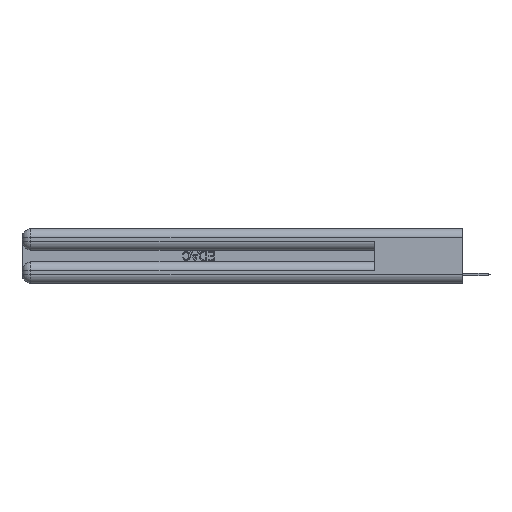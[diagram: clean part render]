
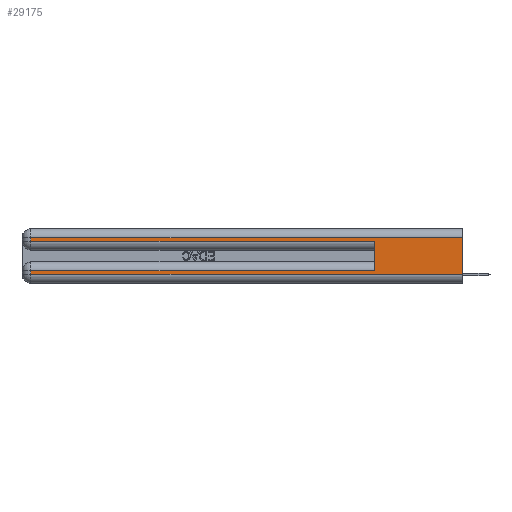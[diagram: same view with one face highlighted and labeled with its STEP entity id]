
A CAD part, left-side view. The second image highlights one B-rep face of the part: STEP entity #29175.
In plain terms, the highlighted planar face has unit normal (-1, 0, 0).
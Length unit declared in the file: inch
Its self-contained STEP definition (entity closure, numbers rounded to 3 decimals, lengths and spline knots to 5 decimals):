
#602 = CARTESIAN_POINT ( 'NONE',  ( 0., 0.6, 0.285 ) ) ;
#2371 = ORIENTED_EDGE ( 'NONE', *, *, #28111, .F. ) ;
#3417 = CARTESIAN_POINT ( 'NONE',  ( 0., 2.94, 0.06 ) ) ;
#3818 = VECTOR ( 'NONE', #21865, 39.37008 ) ;
#4073 = VERTEX_POINT ( 'NONE', #13215 ) ;
#4183 = CARTESIAN_POINT ( 'NONE',  ( 0., 0., 0.085 ) ) ;
#5601 = DIRECTION ( 'NONE',  ( 0., 0., -1. ) ) ;
#5633 = CARTESIAN_POINT ( 'NONE',  ( 0., 2.94, 0.37 ) ) ;
#5733 = VERTEX_POINT ( 'NONE', #23110 ) ;
#6601 = VECTOR ( 'NONE', #24062, 39.37008 ) ;
#7464 = CARTESIAN_POINT ( 'NONE',  ( 0., 2.94, 0.285 ) ) ;
#8403 = DIRECTION ( 'NONE',  ( 0., 0., -1. ) ) ;
#8407 = FACE_OUTER_BOUND ( 'NONE', #9168, .T. ) ;
#8668 = CARTESIAN_POINT ( 'NONE',  ( 0., 2.94, 0.37 ) ) ;
#9168 = EDGE_LOOP ( 'NONE', ( #2371, #9334, #14857, #19345, #15535, #33169, #9845, #17800 ) ) ;
#9334 = ORIENTED_EDGE ( 'NONE', *, *, #15709, .T. ) ;
#9370 = CARTESIAN_POINT ( 'NONE',  ( 0., 0., 0.06 ) ) ;
#9845 = ORIENTED_EDGE ( 'NONE', *, *, #10535, .T. ) ;
#10024 = EDGE_CURVE ( 'NONE', #20692, #19941, #28685, .T. ) ;
#10422 = DIRECTION ( 'NONE',  ( 0., 1., 0. ) ) ;
#10535 = EDGE_CURVE ( 'NONE', #12160, #20692, #29717, .T. ) ;
#10792 = LINE ( 'NONE', #27416, #31409 ) ;
#12160 = VERTEX_POINT ( 'NONE', #34015 ) ;
#13124 = CARTESIAN_POINT ( 'NONE',  ( 0., 0., 0.31 ) ) ;
#13215 = CARTESIAN_POINT ( 'NONE',  ( 0., 0.6, 0.085 ) ) ;
#13992 = DIRECTION ( 'NONE',  ( 1., 0., 0. ) ) ;
#14857 = ORIENTED_EDGE ( 'NONE', *, *, #19500, .T. ) ;
#15257 = CARTESIAN_POINT ( 'NONE',  ( 0., 0., 0.06 ) ) ;
#15535 = ORIENTED_EDGE ( 'NONE', *, *, #27679, .F. ) ;
#15709 = EDGE_CURVE ( 'NONE', #5733, #21085, #35514, .T. ) ;
#16239 = VERTEX_POINT ( 'NONE', #602 ) ;
#16687 = VECTOR ( 'NONE', #23431, 39.37008 ) ;
#17800 = ORIENTED_EDGE ( 'NONE', *, *, #10024, .T. ) ;
#18989 = CARTESIAN_POINT ( 'NONE',  ( 0., 0., 0.285 ) ) ;
#19064 = CARTESIAN_POINT ( 'NONE',  ( 0., 0., 0.37 ) ) ;
#19345 = ORIENTED_EDGE ( 'NONE', *, *, #31973, .T. ) ;
#19500 = EDGE_CURVE ( 'NONE', #21085, #34654, #19866, .T. ) ;
#19866 = LINE ( 'NONE', #8668, #20342 ) ;
#19941 = VERTEX_POINT ( 'NONE', #15257 ) ;
#20342 = VECTOR ( 'NONE', #5601, 39.37008 ) ;
#20521 = AXIS2_PLACEMENT_3D ( 'NONE', #19064, #13992, #30086 ) ;
#20692 = VERTEX_POINT ( 'NONE', #3417 ) ;
#21085 = VERTEX_POINT ( 'NONE', #30675 ) ;
#21805 = DIRECTION ( 'NONE',  ( 0., 0., 1. ) ) ;
#21865 = DIRECTION ( 'NONE',  ( 0., -1., 0. ) ) ;
#22110 = CARTESIAN_POINT ( 'NONE',  ( 0., 0., 0.37 ) ) ;
#22214 = LINE ( 'NONE', #18989, #3818 ) ;
#23110 = CARTESIAN_POINT ( 'NONE',  ( 0., 0., 0.31 ) ) ;
#23431 = DIRECTION ( 'NONE',  ( 0., -1., 0. ) ) ;
#23634 = EDGE_CURVE ( 'NONE', #4073, #12160, #26063, .T. ) ;
#24062 = DIRECTION ( 'NONE',  ( 0., 1., 0. ) ) ;
#24650 = PLANE ( 'NONE',  #20521 ) ;
#24822 = LINE ( 'NONE', #22110, #33741 ) ;
#26063 = LINE ( 'NONE', #4183, #6601 ) ;
#27416 = CARTESIAN_POINT ( 'NONE',  ( 0., 0.6, 0.145 ) ) ;
#27679 = EDGE_CURVE ( 'NONE', #4073, #16239, #10792, .T. ) ;
#28111 = EDGE_CURVE ( 'NONE', #5733, #19941, #24822, .T. ) ;
#28302 = VECTOR ( 'NONE', #10422, 39.37008 ) ;
#28685 = LINE ( 'NONE', #9370, #16687 ) ;
#29175 = ADVANCED_FACE ( 'NONE', ( #8407 ), #24650, .F. ) ;
#29717 = LINE ( 'NONE', #5633, #34708 ) ;
#30086 = DIRECTION ( 'NONE',  ( 0., 0., -1. ) ) ;
#30554 = DIRECTION ( 'NONE',  ( 0., 0., -1. ) ) ;
#30675 = CARTESIAN_POINT ( 'NONE',  ( 0., 2.94, 0.31 ) ) ;
#31409 = VECTOR ( 'NONE', #21805, 39.37008 ) ;
#31973 = EDGE_CURVE ( 'NONE', #34654, #16239, #22214, .T. ) ;
#33169 = ORIENTED_EDGE ( 'NONE', *, *, #23634, .T. ) ;
#33741 = VECTOR ( 'NONE', #8403, 39.37008 ) ;
#34015 = CARTESIAN_POINT ( 'NONE',  ( 0., 2.94, 0.085 ) ) ;
#34654 = VERTEX_POINT ( 'NONE', #7464 ) ;
#34708 = VECTOR ( 'NONE', #30554, 39.37008 ) ;
#35514 = LINE ( 'NONE', #13124, #28302 ) ;
